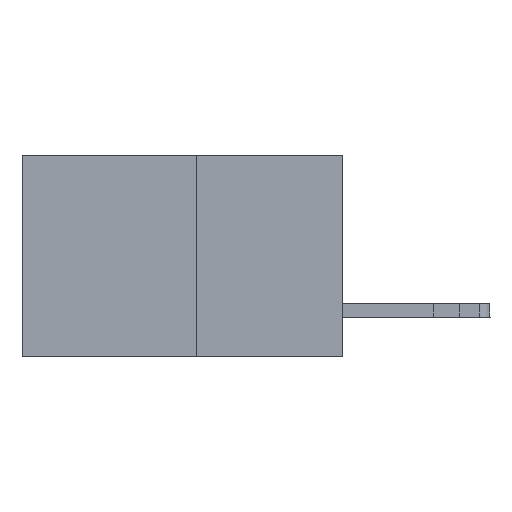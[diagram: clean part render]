
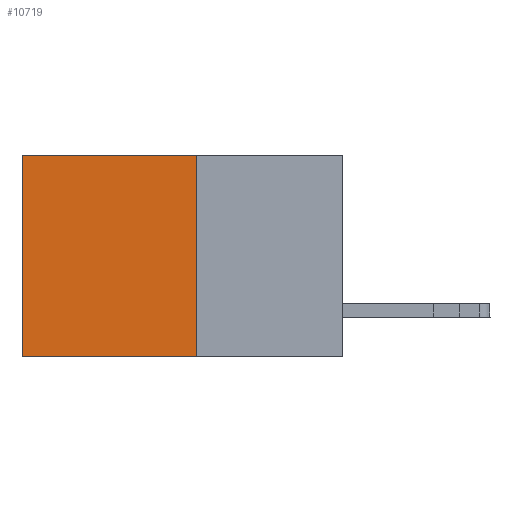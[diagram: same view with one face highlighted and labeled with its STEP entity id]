
A CAD part, left-side view. The second image highlights one B-rep face of the part: STEP entity #10719.
In plain terms, the highlighted planar face has unit normal (-1, 0, 0).
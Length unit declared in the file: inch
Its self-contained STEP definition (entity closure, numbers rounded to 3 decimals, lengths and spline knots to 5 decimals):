
#551 = VERTEX_POINT ( 'NONE', #2935 ) ;
#566 = DIRECTION ( 'NONE',  ( 0., 1., 0. ) ) ;
#766 = DIRECTION ( 'NONE',  ( 0., 0., -1. ) ) ;
#2917 = CARTESIAN_POINT ( 'NONE',  ( 0.277, 0.27, -0.37 ) ) ;
#2935 = CARTESIAN_POINT ( 'NONE',  ( 0.277, 0.59, -0.37 ) ) ;
#3287 = FACE_OUTER_BOUND ( 'NONE', #24424, .T. ) ;
#3588 = ORIENTED_EDGE ( 'NONE', *, *, #21023, .T. ) ;
#4260 = CARTESIAN_POINT ( 'NONE',  ( 0.277, 0.27, 0. ) ) ;
#4729 = VECTOR ( 'NONE', #14387, 39.37008 ) ;
#5327 = DIRECTION ( 'NONE',  ( 0., 0., -1. ) ) ;
#5362 = EDGE_CURVE ( 'NONE', #12125, #551, #22645, .T. ) ;
#5584 = CARTESIAN_POINT ( 'NONE',  ( 0.277, 0.59, 0. ) ) ;
#5775 = VECTOR ( 'NONE', #14382, 39.37008 ) ;
#7256 = VERTEX_POINT ( 'NONE', #5584 ) ;
#7315 = ORIENTED_EDGE ( 'NONE', *, *, #22340, .F. ) ;
#8408 = CARTESIAN_POINT ( 'NONE',  ( 0.277, 0.59, -0.37 ) ) ;
#8928 = VECTOR ( 'NONE', #766, 39.37008 ) ;
#10719 = ADVANCED_FACE ( 'NONE', ( #3287 ), #11430, .F. ) ;
#11430 = PLANE ( 'NONE',  #18002 ) ;
#12125 = VERTEX_POINT ( 'NONE', #18723 ) ;
#13565 = EDGE_CURVE ( 'NONE', #15916, #7256, #21827, .T. ) ;
#14262 = LINE ( 'NONE', #8408, #4729 ) ;
#14382 = DIRECTION ( 'NONE',  ( 0., 1., 0. ) ) ;
#14387 = DIRECTION ( 'NONE',  ( 0., 0., -1. ) ) ;
#15004 = DIRECTION ( 'NONE',  ( 1., 0., 0. ) ) ;
#15916 = VERTEX_POINT ( 'NONE', #19756 ) ;
#16508 = ORIENTED_EDGE ( 'NONE', *, *, #13565, .T. ) ;
#16786 = CARTESIAN_POINT ( 'NONE',  ( 0.277, 0.27, -0.37 ) ) ;
#17856 = VECTOR ( 'NONE', #566, 39.37008 ) ;
#18002 = AXIS2_PLACEMENT_3D ( 'NONE', #16786, #15004, #5327 ) ;
#18085 = LINE ( 'NONE', #18208, #8928 ) ;
#18208 = CARTESIAN_POINT ( 'NONE',  ( 0.277, 0.27, -0.37 ) ) ;
#18723 = CARTESIAN_POINT ( 'NONE',  ( 0.277, 0.27, -0.37 ) ) ;
#19756 = CARTESIAN_POINT ( 'NONE',  ( 0.277, 0.27, 0. ) ) ;
#20190 = ORIENTED_EDGE ( 'NONE', *, *, #5362, .F. ) ;
#21023 = EDGE_CURVE ( 'NONE', #7256, #551, #14262, .T. ) ;
#21827 = LINE ( 'NONE', #4260, #17856 ) ;
#22340 = EDGE_CURVE ( 'NONE', #15916, #12125, #18085, .T. ) ;
#22645 = LINE ( 'NONE', #2917, #5775 ) ;
#24424 = EDGE_LOOP ( 'NONE', ( #3588, #20190, #7315, #16508 ) ) ;
